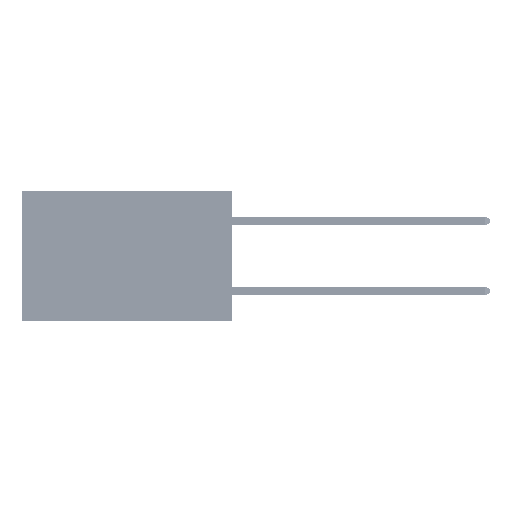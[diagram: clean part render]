
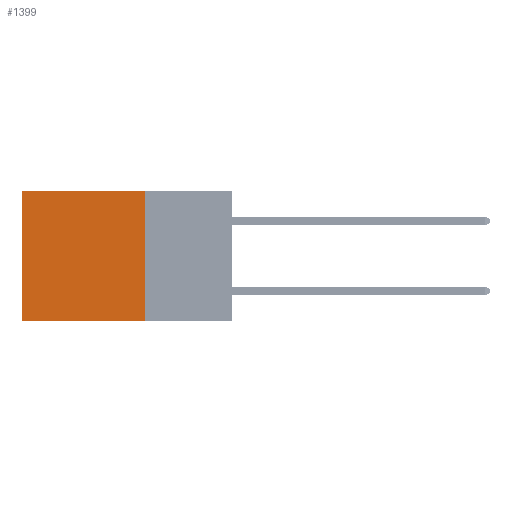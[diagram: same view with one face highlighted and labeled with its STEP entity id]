
A CAD part, left-side view. The second image highlights one B-rep face of the part: STEP entity #1399.
In plain terms, the highlighted planar face has unit normal (-1, 0, 0).
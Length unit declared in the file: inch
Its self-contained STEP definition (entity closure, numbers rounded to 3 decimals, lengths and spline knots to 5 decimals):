
#648 = VECTOR ( 'NONE', #46977, 39.37008 ) ;
#1128 = ORIENTED_EDGE ( 'NONE', *, *, #14105, .T. ) ;
#1154 = AXIS2_PLACEMENT_3D ( 'NONE', #22486, #26692, #50668 ) ;
#1399 = ADVANCED_FACE ( 'NONE', ( #36179 ), #18452, .F. ) ;
#2998 = ORIENTED_EDGE ( 'NONE', *, *, #17129, .F. ) ;
#4373 = VECTOR ( 'NONE', #4969, 39.37008 ) ;
#4969 = DIRECTION ( 'NONE',  ( 0., 1., 0. ) ) ;
#6801 = VERTEX_POINT ( 'NONE', #11289 ) ;
#11289 = CARTESIAN_POINT ( 'NONE',  ( 0.2875, 0.25, -0.37 ) ) ;
#14105 = EDGE_CURVE ( 'NONE', #48360, #48363, #33901, .T. ) ;
#15129 = ORIENTED_EDGE ( 'NONE', *, *, #31115, .T. ) ;
#17129 = EDGE_CURVE ( 'NONE', #6801, #48363, #42790, .T. ) ;
#17996 = DIRECTION ( 'NONE',  ( 0., 0., -1. ) ) ;
#18205 = DIRECTION ( 'NONE',  ( 0., 1., 0. ) ) ;
#18347 = CARTESIAN_POINT ( 'NONE',  ( 0.2875, 0.6, 0. ) ) ;
#18452 = PLANE ( 'NONE',  #1154 ) ;
#19950 = EDGE_LOOP ( 'NONE', ( #1128, #2998, #49057, #15129 ) ) ;
#21196 = CARTESIAN_POINT ( 'NONE',  ( 0.2875, 0.25, -0.37 ) ) ;
#22486 = CARTESIAN_POINT ( 'NONE',  ( 0.2875, 0.25, 0. ) ) ;
#26073 = VERTEX_POINT ( 'NONE', #32333 ) ;
#26692 = DIRECTION ( 'NONE',  ( 1., 0., 0. ) ) ;
#31115 = EDGE_CURVE ( 'NONE', #26073, #48360, #40334, .T. ) ;
#31368 = VECTOR ( 'NONE', #17996, 39.37008 ) ;
#32333 = CARTESIAN_POINT ( 'NONE',  ( 0.2875, 0.25, 0. ) ) ;
#32377 = CARTESIAN_POINT ( 'NONE',  ( 0.2875, 0.6, 0. ) ) ;
#33901 = LINE ( 'NONE', #18347, #31368 ) ;
#36179 = FACE_OUTER_BOUND ( 'NONE', #19950, .T. ) ;
#38843 = CARTESIAN_POINT ( 'NONE',  ( 0.2875, 0.25, 0. ) ) ;
#40334 = LINE ( 'NONE', #42981, #41588 ) ;
#40940 = LINE ( 'NONE', #38843, #648 ) ;
#41588 = VECTOR ( 'NONE', #18205, 39.37008 ) ;
#42790 = LINE ( 'NONE', #21196, #4373 ) ;
#42981 = CARTESIAN_POINT ( 'NONE',  ( 0.2875, 0.25, 0. ) ) ;
#43995 = CARTESIAN_POINT ( 'NONE',  ( 0.2875, 0.6, -0.37 ) ) ;
#46977 = DIRECTION ( 'NONE',  ( 0., 0., -1. ) ) ;
#48360 = VERTEX_POINT ( 'NONE', #32377 ) ;
#48363 = VERTEX_POINT ( 'NONE', #43995 ) ;
#48704 = EDGE_CURVE ( 'NONE', #26073, #6801, #40940, .T. ) ;
#49057 = ORIENTED_EDGE ( 'NONE', *, *, #48704, .F. ) ;
#50668 = DIRECTION ( 'NONE',  ( 0., 0., -1. ) ) ;
